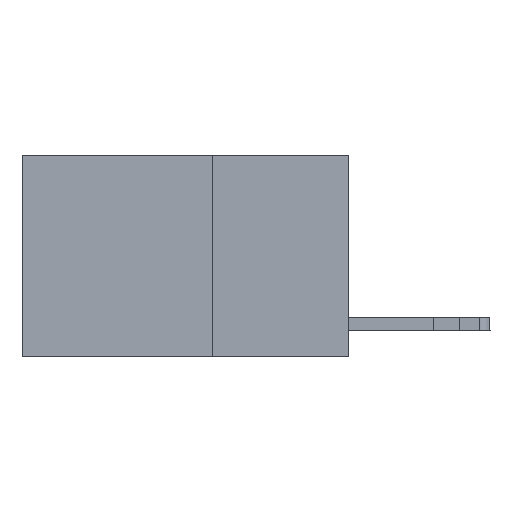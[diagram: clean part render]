
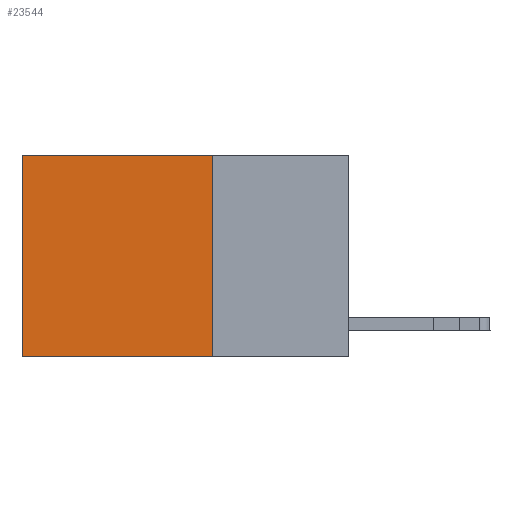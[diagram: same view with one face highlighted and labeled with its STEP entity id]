
A CAD part, left-side view. The second image highlights one B-rep face of the part: STEP entity #23544.
In plain terms, the highlighted planar face has unit normal (-1, 0, 0).
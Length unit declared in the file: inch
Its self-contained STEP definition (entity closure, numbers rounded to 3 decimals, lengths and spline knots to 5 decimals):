
#476 = CARTESIAN_POINT ( 'NONE',  ( 0.2625, 0.6, 0. ) ) ;
#664 = VECTOR ( 'NONE', #18111, 39.37008 ) ;
#736 = VECTOR ( 'NONE', #9002, 39.37008 ) ;
#1086 = DIRECTION ( 'NONE',  ( 0., 1., 0. ) ) ;
#1975 = VERTEX_POINT ( 'NONE', #2213 ) ;
#2213 = CARTESIAN_POINT ( 'NONE',  ( 0.2625, 0.6, 0. ) ) ;
#2961 = LINE ( 'NONE', #10566, #18373 ) ;
#4918 = DIRECTION ( 'NONE',  ( 1., 0., 0. ) ) ;
#8168 = VECTOR ( 'NONE', #23721, 39.37008 ) ;
#9002 = DIRECTION ( 'NONE',  ( 0., 0., -1. ) ) ;
#9008 = CARTESIAN_POINT ( 'NONE',  ( 0.2625, 0.25, 0. ) ) ;
#10150 = ORIENTED_EDGE ( 'NONE', *, *, #20138, .T. ) ;
#10204 = LINE ( 'NONE', #476, #664 ) ;
#10566 = CARTESIAN_POINT ( 'NONE',  ( 0.2625, 0.25, 0. ) ) ;
#10928 = EDGE_CURVE ( 'NONE', #15306, #17835, #24209, .T. ) ;
#11487 = EDGE_CURVE ( 'NONE', #15306, #1975, #2961, .T. ) ;
#12318 = ORIENTED_EDGE ( 'NONE', *, *, #11487, .T. ) ;
#12348 = EDGE_LOOP ( 'NONE', ( #10150, #13708, #13791, #12318 ) ) ;
#12829 = VERTEX_POINT ( 'NONE', #14862 ) ;
#12891 = FACE_OUTER_BOUND ( 'NONE', #12348, .T. ) ;
#13708 = ORIENTED_EDGE ( 'NONE', *, *, #17958, .F. ) ;
#13791 = ORIENTED_EDGE ( 'NONE', *, *, #10928, .F. ) ;
#14261 = CARTESIAN_POINT ( 'NONE',  ( 0.2625, 0.25, -0.37 ) ) ;
#14862 = CARTESIAN_POINT ( 'NONE',  ( 0.2625, 0.6, -0.37 ) ) ;
#15306 = VERTEX_POINT ( 'NONE', #20883 ) ;
#16021 = LINE ( 'NONE', #14261, #8168 ) ;
#16513 = PLANE ( 'NONE',  #21174 ) ;
#17835 = VERTEX_POINT ( 'NONE', #18812 ) ;
#17958 = EDGE_CURVE ( 'NONE', #17835, #12829, #16021, .T. ) ;
#18111 = DIRECTION ( 'NONE',  ( 0., 0., -1. ) ) ;
#18373 = VECTOR ( 'NONE', #1086, 39.37008 ) ;
#18812 = CARTESIAN_POINT ( 'NONE',  ( 0.2625, 0.25, -0.37 ) ) ;
#20138 = EDGE_CURVE ( 'NONE', #1975, #12829, #10204, .T. ) ;
#20308 = DIRECTION ( 'NONE',  ( 0., 0., -1. ) ) ;
#20883 = CARTESIAN_POINT ( 'NONE',  ( 0.2625, 0.25, 0. ) ) ;
#21174 = AXIS2_PLACEMENT_3D ( 'NONE', #9008, #4918, #20308 ) ;
#22102 = CARTESIAN_POINT ( 'NONE',  ( 0.2625, 0.25, 0. ) ) ;
#23544 = ADVANCED_FACE ( 'NONE', ( #12891 ), #16513, .F. ) ;
#23721 = DIRECTION ( 'NONE',  ( 0., 1., 0. ) ) ;
#24209 = LINE ( 'NONE', #22102, #736 ) ;
